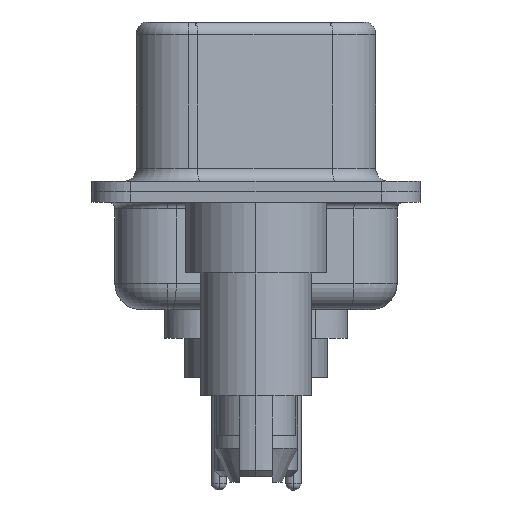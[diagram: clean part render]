
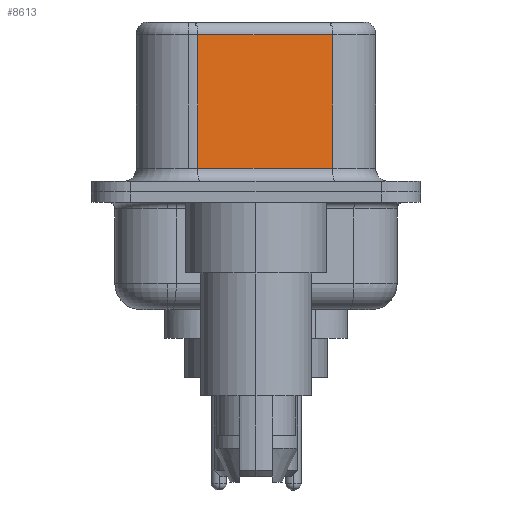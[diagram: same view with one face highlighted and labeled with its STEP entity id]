
A CAD part, left-side view. The second image highlights one B-rep face of the part: STEP entity #8613.
In plain terms, the highlighted planar face has unit normal (-0.985, -0.174, 0).
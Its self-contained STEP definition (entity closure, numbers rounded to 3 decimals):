
#51 = CARTESIAN_POINT ( 'NONE',  ( 4.58, -2.927, 6.02 ) ) ;
#2137 = ORIENTED_EDGE ( 'NONE', *, *, #19271, .T. ) ;
#2757 = PLANE ( 'NONE',  #9115 ) ;
#3012 = LINE ( 'NONE', #21590, #16712 ) ;
#4258 = VERTEX_POINT ( 'NONE', #7707 ) ;
#4302 = VECTOR ( 'NONE', #15373, 1000. ) ;
#4419 = CARTESIAN_POINT ( 'NONE',  ( 4.58, -2.927, 6.52 ) ) ;
#4566 = VERTEX_POINT ( 'NONE', #51 ) ;
#4610 = DIRECTION ( 'NONE',  ( -0.174, 0.985, 0. ) ) ;
#5156 = EDGE_LOOP ( 'NONE', ( #21437, #2137, #14268, #23771 ) ) ;
#5645 = VECTOR ( 'NONE', #6896, 1000. ) ;
#6448 = CARTESIAN_POINT ( 'NONE',  ( 4.58, -2.927, 0.9 ) ) ;
#6896 = DIRECTION ( 'NONE',  ( 0., 0., -1. ) ) ;
#7707 = CARTESIAN_POINT ( 'NONE',  ( 3.67, 2.233, 6.02 ) ) ;
#8517 = DIRECTION ( 'NONE',  ( -0.174, 0.985, 0. ) ) ;
#8536 = LINE ( 'NONE', #17261, #4302 ) ;
#8613 = ADVANCED_FACE ( 'NONE', ( #18656 ), #2757, .F. ) ;
#9115 = AXIS2_PLACEMENT_3D ( 'NONE', #19402, #15779, #4610 ) ;
#10865 = VECTOR ( 'NONE', #17486, 1000. ) ;
#11317 = EDGE_CURVE ( 'NONE', #4258, #14325, #20013, .T. ) ;
#13716 = EDGE_CURVE ( 'NONE', #4566, #18833, #20775, .T. ) ;
#14268 = ORIENTED_EDGE ( 'NONE', *, *, #11317, .T. ) ;
#14325 = VERTEX_POINT ( 'NONE', #17379 ) ;
#15250 = EDGE_CURVE ( 'NONE', #14325, #18833, #8536, .T. ) ;
#15373 = DIRECTION ( 'NONE',  ( 0.174, -0.985, 0. ) ) ;
#15779 = DIRECTION ( 'NONE',  ( 0.985, 0.174, 0. ) ) ;
#16712 = VECTOR ( 'NONE', #8517, 1000. ) ;
#17261 = CARTESIAN_POINT ( 'NONE',  ( 4.58, -2.927, 0.9 ) ) ;
#17379 = CARTESIAN_POINT ( 'NONE',  ( 3.67, 2.233, 0.9 ) ) ;
#17486 = DIRECTION ( 'NONE',  ( 0., 0., -1. ) ) ;
#18127 = CARTESIAN_POINT ( 'NONE',  ( 3.67, 2.233, 6.52 ) ) ;
#18656 = FACE_OUTER_BOUND ( 'NONE', #5156, .T. ) ;
#18833 = VERTEX_POINT ( 'NONE', #6448 ) ;
#19271 = EDGE_CURVE ( 'NONE', #4566, #4258, #3012, .T. ) ;
#19402 = CARTESIAN_POINT ( 'NONE',  ( 4.58, -2.927, 6.52 ) ) ;
#20013 = LINE ( 'NONE', #18127, #5645 ) ;
#20775 = LINE ( 'NONE', #4419, #10865 ) ;
#21437 = ORIENTED_EDGE ( 'NONE', *, *, #13716, .F. ) ;
#21590 = CARTESIAN_POINT ( 'NONE',  ( 4.58, -2.927, 6.02 ) ) ;
#23771 = ORIENTED_EDGE ( 'NONE', *, *, #15250, .T. ) ;
